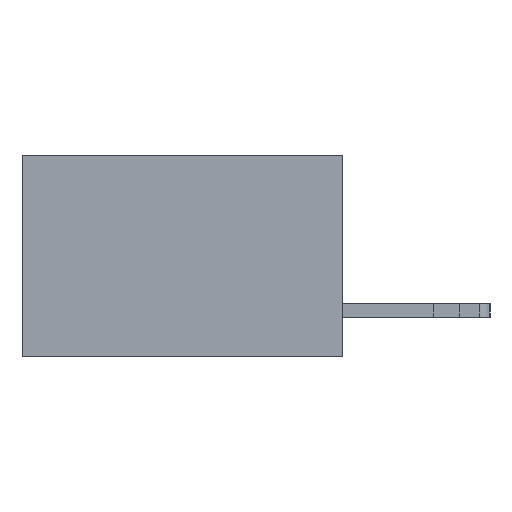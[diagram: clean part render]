
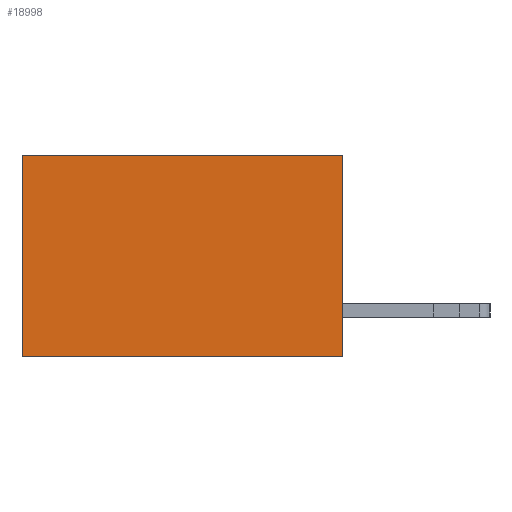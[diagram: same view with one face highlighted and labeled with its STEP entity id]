
A CAD part, left-side view. The second image highlights one B-rep face of the part: STEP entity #18998.
In plain terms, the highlighted planar face has unit normal (-1, 0, 0).
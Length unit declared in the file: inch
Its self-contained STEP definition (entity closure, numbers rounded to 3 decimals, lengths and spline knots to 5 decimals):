
#487 = ORIENTED_EDGE ( 'NONE', *, *, #1985, .T. ) ;
#710 = VERTEX_POINT ( 'NONE', #1591 ) ;
#1122 = VERTEX_POINT ( 'NONE', #17186 ) ;
#1458 = FACE_OUTER_BOUND ( 'NONE', #18833, .T. ) ;
#1591 = CARTESIAN_POINT ( 'NONE',  ( 0.277, 0.59, -0.37 ) ) ;
#1985 = EDGE_CURVE ( 'NONE', #9089, #710, #22416, .T. ) ;
#2679 = EDGE_CURVE ( 'NONE', #9950, #1122, #16874, .T. ) ;
#4300 = DIRECTION ( 'NONE',  ( 1., 0., 0. ) ) ;
#6798 = AXIS2_PLACEMENT_3D ( 'NONE', #21653, #4300, #19508 ) ;
#6823 = DIRECTION ( 'NONE',  ( 0., 0., -1. ) ) ;
#6984 = CARTESIAN_POINT ( 'NONE',  ( 0.277, 0.59, 0. ) ) ;
#7720 = LINE ( 'NONE', #22297, #18538 ) ;
#8511 = CARTESIAN_POINT ( 'NONE',  ( 0.277, 0., 0. ) ) ;
#9089 = VERTEX_POINT ( 'NONE', #6984 ) ;
#9658 = LINE ( 'NONE', #8511, #14760 ) ;
#9950 = VERTEX_POINT ( 'NONE', #14719 ) ;
#10679 = DIRECTION ( 'NONE',  ( 0., 1., 0. ) ) ;
#11416 = DIRECTION ( 'NONE',  ( 0., 1., 0. ) ) ;
#11542 = ORIENTED_EDGE ( 'NONE', *, *, #2679, .F. ) ;
#13549 = EDGE_CURVE ( 'NONE', #1122, #710, #7720, .T. ) ;
#14719 = CARTESIAN_POINT ( 'NONE',  ( 0.277, 0., 0. ) ) ;
#14760 = VECTOR ( 'NONE', #10679, 39.37008 ) ;
#14770 = CARTESIAN_POINT ( 'NONE',  ( 0.277, 0.59, -0.37 ) ) ;
#15958 = ORIENTED_EDGE ( 'NONE', *, *, #13549, .F. ) ;
#16193 = VECTOR ( 'NONE', #6823, 39.37008 ) ;
#16586 = VECTOR ( 'NONE', #25299, 39.37008 ) ;
#16874 = LINE ( 'NONE', #19505, #16193 ) ;
#17186 = CARTESIAN_POINT ( 'NONE',  ( 0.277, 0., -0.37 ) ) ;
#17325 = PLANE ( 'NONE',  #6798 ) ;
#18538 = VECTOR ( 'NONE', #11416, 39.37008 ) ;
#18833 = EDGE_LOOP ( 'NONE', ( #487, #15958, #11542, #19363 ) ) ;
#18998 = ADVANCED_FACE ( 'NONE', ( #1458 ), #17325, .F. ) ;
#19363 = ORIENTED_EDGE ( 'NONE', *, *, #25421, .T. ) ;
#19505 = CARTESIAN_POINT ( 'NONE',  ( 0.277, 0., -0.37 ) ) ;
#19508 = DIRECTION ( 'NONE',  ( 0., 0., -1. ) ) ;
#21653 = CARTESIAN_POINT ( 'NONE',  ( 0.277, 0., -0.37 ) ) ;
#22297 = CARTESIAN_POINT ( 'NONE',  ( 0.277, 0., -0.37 ) ) ;
#22416 = LINE ( 'NONE', #14770, #16586 ) ;
#25299 = DIRECTION ( 'NONE',  ( 0., 0., -1. ) ) ;
#25421 = EDGE_CURVE ( 'NONE', #9950, #9089, #9658, .T. ) ;
